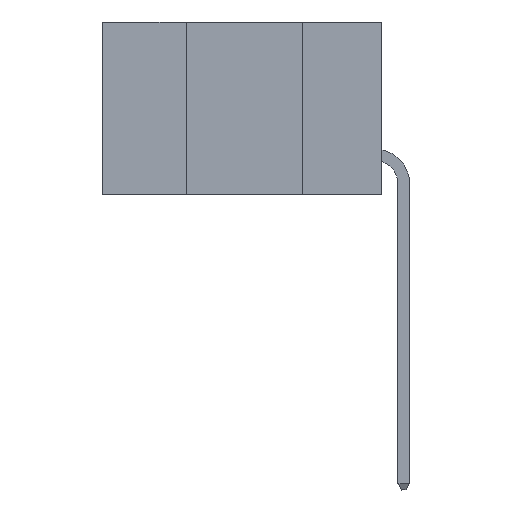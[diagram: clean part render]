
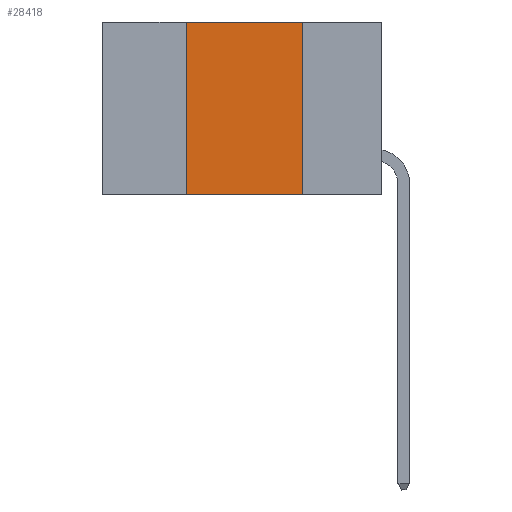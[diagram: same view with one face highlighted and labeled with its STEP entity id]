
A CAD part, left-side view. The second image highlights one B-rep face of the part: STEP entity #28418.
In plain terms, the highlighted planar face has unit normal (-1, 0, 0).
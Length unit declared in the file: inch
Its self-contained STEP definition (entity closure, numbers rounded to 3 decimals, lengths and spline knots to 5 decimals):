
#703 = EDGE_CURVE ( 'NONE', #15867, #17594, #7922, .T. ) ;
#1628 = CARTESIAN_POINT ( 'NONE',  ( 0., 0.17, -0.37 ) ) ;
#1698 = CARTESIAN_POINT ( 'NONE',  ( 0., 0.42, 0. ) ) ;
#3361 = EDGE_CURVE ( 'NONE', #17594, #10609, #25395, .T. ) ;
#6167 = VECTOR ( 'NONE', #26452, 39.37008 ) ;
#6577 = CARTESIAN_POINT ( 'NONE',  ( 0., 0.6, 0. ) ) ;
#6736 = CARTESIAN_POINT ( 'NONE',  ( 0., 0.42, 0. ) ) ;
#6815 = DIRECTION ( 'NONE',  ( 1., 0., 0. ) ) ;
#6844 = LINE ( 'NONE', #16847, #9701 ) ;
#7922 = LINE ( 'NONE', #1698, #6167 ) ;
#7989 = DIRECTION ( 'NONE',  ( 0., -1., 0. ) ) ;
#8245 = AXIS2_PLACEMENT_3D ( 'NONE', #19024, #6815, #17955 ) ;
#9556 = CARTESIAN_POINT ( 'NONE',  ( 0., 0.17, 0. ) ) ;
#9701 = VECTOR ( 'NONE', #7989, 39.37008 ) ;
#9860 = ORIENTED_EDGE ( 'NONE', *, *, #25563, .F. ) ;
#10609 = VERTEX_POINT ( 'NONE', #22394 ) ;
#15199 = FACE_OUTER_BOUND ( 'NONE', #27077, .T. ) ;
#15388 = VECTOR ( 'NONE', #25475, 39.37008 ) ;
#15867 = VERTEX_POINT ( 'NONE', #19324 ) ;
#15911 = PLANE ( 'NONE',  #8245 ) ;
#16847 = CARTESIAN_POINT ( 'NONE',  ( 0., 0.6, -0.37 ) ) ;
#17594 = VERTEX_POINT ( 'NONE', #6736 ) ;
#17955 = DIRECTION ( 'NONE',  ( 0., 0., -1. ) ) ;
#18388 = ORIENTED_EDGE ( 'NONE', *, *, #703, .F. ) ;
#19024 = CARTESIAN_POINT ( 'NONE',  ( 0., 0.6, 0. ) ) ;
#19324 = CARTESIAN_POINT ( 'NONE',  ( 0., 0.42, -0.37 ) ) ;
#21335 = LINE ( 'NONE', #9556, #15388 ) ;
#22092 = ORIENTED_EDGE ( 'NONE', *, *, #24921, .T. ) ;
#22394 = CARTESIAN_POINT ( 'NONE',  ( 0., 0.17, 0. ) ) ;
#22483 = DIRECTION ( 'NONE',  ( 0., -1., 0. ) ) ;
#24921 = EDGE_CURVE ( 'NONE', #15867, #29336, #6844, .T. ) ;
#25395 = LINE ( 'NONE', #6577, #29001 ) ;
#25475 = DIRECTION ( 'NONE',  ( 0., 0., -1. ) ) ;
#25563 = EDGE_CURVE ( 'NONE', #10609, #29336, #21335, .T. ) ;
#26452 = DIRECTION ( 'NONE',  ( 0., 0., 1. ) ) ;
#27077 = EDGE_LOOP ( 'NONE', ( #9860, #28073, #18388, #22092 ) ) ;
#28073 = ORIENTED_EDGE ( 'NONE', *, *, #3361, .F. ) ;
#28418 = ADVANCED_FACE ( 'NONE', ( #15199 ), #15911, .F. ) ;
#29001 = VECTOR ( 'NONE', #22483, 39.37008 ) ;
#29336 = VERTEX_POINT ( 'NONE', #1628 ) ;
